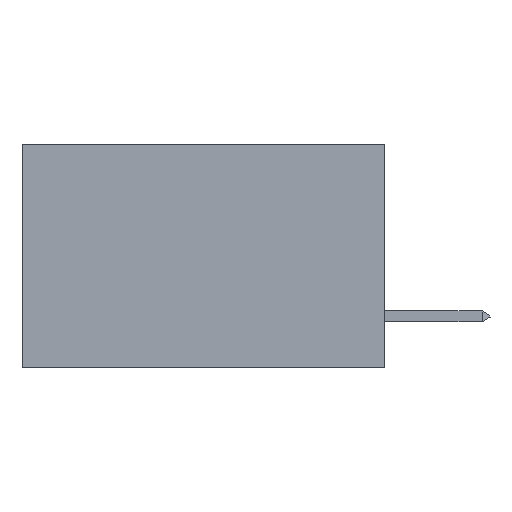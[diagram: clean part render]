
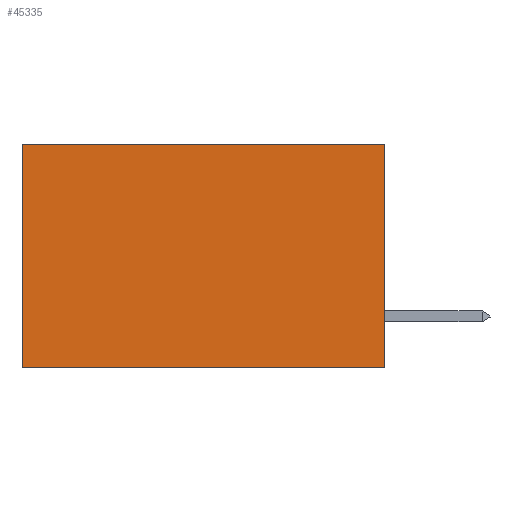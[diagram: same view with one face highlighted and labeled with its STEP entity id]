
A CAD part, left-side view. The second image highlights one B-rep face of the part: STEP entity #45335.
In plain terms, the highlighted planar face has unit normal (-1, 0, 0).
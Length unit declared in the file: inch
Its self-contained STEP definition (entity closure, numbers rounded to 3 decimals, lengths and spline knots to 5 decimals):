
#1219 = ORIENTED_EDGE ( 'NONE', *, *, #2423, .F. ) ;
#1349 = CARTESIAN_POINT ( 'NONE',  ( 0.2875, 0., 0. ) ) ;
#2423 = EDGE_CURVE ( 'NONE', #13217, #42229, #22733, .T. ) ;
#5738 = DIRECTION ( 'NONE',  ( 0., 0., -1. ) ) ;
#9167 = DIRECTION ( 'NONE',  ( 0., 1., 0. ) ) ;
#11026 = EDGE_LOOP ( 'NONE', ( #36108, #1219, #39388, #28871 ) ) ;
#13217 = VERTEX_POINT ( 'NONE', #42614 ) ;
#13298 = VECTOR ( 'NONE', #45602, 39.37008 ) ;
#14205 = EDGE_CURVE ( 'NONE', #27034, #42396, #17718, .T. ) ;
#15395 = LINE ( 'NONE', #31887, #32802 ) ;
#17718 = LINE ( 'NONE', #41950, #34031 ) ;
#17786 = AXIS2_PLACEMENT_3D ( 'NONE', #27065, #41922, #5738 ) ;
#18259 = EDGE_CURVE ( 'NONE', #27034, #13217, #38664, .T. ) ;
#19385 = FACE_OUTER_BOUND ( 'NONE', #11026, .T. ) ;
#20308 = CARTESIAN_POINT ( 'NONE',  ( 0.2875, 0., 0. ) ) ;
#22733 = LINE ( 'NONE', #31184, #13298 ) ;
#23620 = CARTESIAN_POINT ( 'NONE',  ( 0.2875, 0.6, -0.37 ) ) ;
#26656 = CARTESIAN_POINT ( 'NONE',  ( 0.2875, 0.6, 0. ) ) ;
#27034 = VERTEX_POINT ( 'NONE', #1349 ) ;
#27065 = CARTESIAN_POINT ( 'NONE',  ( 0.2875, 0., 0. ) ) ;
#28871 = ORIENTED_EDGE ( 'NONE', *, *, #14205, .T. ) ;
#29641 = VECTOR ( 'NONE', #45533, 39.37008 ) ;
#31184 = CARTESIAN_POINT ( 'NONE',  ( 0.2875, 0., -0.37 ) ) ;
#31887 = CARTESIAN_POINT ( 'NONE',  ( 0.2875, 0.6, 0. ) ) ;
#32029 = DIRECTION ( 'NONE',  ( 0., 0., -1. ) ) ;
#32802 = VECTOR ( 'NONE', #32029, 39.37008 ) ;
#34031 = VECTOR ( 'NONE', #9167, 39.37008 ) ;
#36108 = ORIENTED_EDGE ( 'NONE', *, *, #45942, .T. ) ;
#38664 = LINE ( 'NONE', #20308, #29641 ) ;
#39388 = ORIENTED_EDGE ( 'NONE', *, *, #18259, .F. ) ;
#41922 = DIRECTION ( 'NONE',  ( 1., 0., 0. ) ) ;
#41950 = CARTESIAN_POINT ( 'NONE',  ( 0.2875, 0., 0. ) ) ;
#42229 = VERTEX_POINT ( 'NONE', #23620 ) ;
#42396 = VERTEX_POINT ( 'NONE', #26656 ) ;
#42614 = CARTESIAN_POINT ( 'NONE',  ( 0.2875, 0., -0.37 ) ) ;
#44909 = PLANE ( 'NONE',  #17786 ) ;
#45335 = ADVANCED_FACE ( 'NONE', ( #19385 ), #44909, .F. ) ;
#45533 = DIRECTION ( 'NONE',  ( 0., 0., -1. ) ) ;
#45602 = DIRECTION ( 'NONE',  ( 0., 1., 0. ) ) ;
#45942 = EDGE_CURVE ( 'NONE', #42396, #42229, #15395, .T. ) ;
